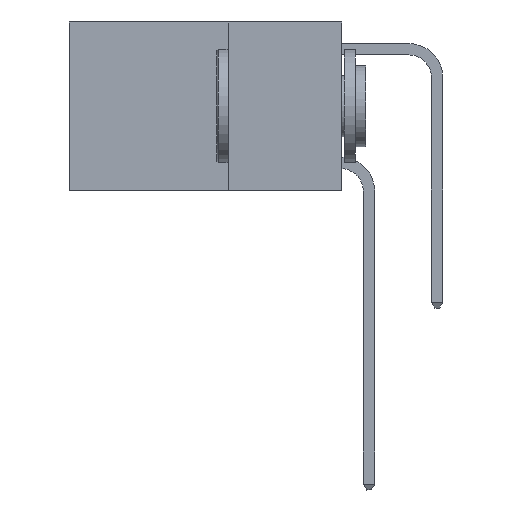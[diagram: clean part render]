
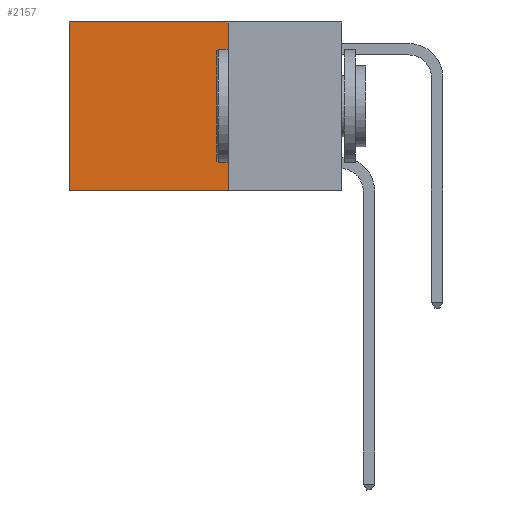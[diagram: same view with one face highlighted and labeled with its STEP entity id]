
A CAD part, left-side view. The second image highlights one B-rep face of the part: STEP entity #2157.
In plain terms, the highlighted planar face has unit normal (-1, 0, 0).
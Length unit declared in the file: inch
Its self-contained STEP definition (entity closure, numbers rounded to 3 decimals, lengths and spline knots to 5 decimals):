
#195 = LINE ( 'NONE', #2769, #5230 ) ;
#414 = ORIENTED_EDGE ( 'NONE', *, *, #4275, .F. ) ;
#1309 = LINE ( 'NONE', #2766, #7239 ) ;
#1412 = DIRECTION ( 'NONE',  ( 0., 0., -1. ) ) ;
#1639 = DIRECTION ( 'NONE',  ( 0., 0., -1. ) ) ;
#1798 = FACE_OUTER_BOUND ( 'NONE', #3617, .T. ) ;
#1962 = DIRECTION ( 'NONE',  ( 0., 0., -1. ) ) ;
#2157 = ADVANCED_FACE ( 'NONE', ( #1798 ), #5561, .F. ) ;
#2766 = CARTESIAN_POINT ( 'NONE',  ( 0.2625, 0.25, -0.37 ) ) ;
#2769 = CARTESIAN_POINT ( 'NONE',  ( 0.2625, 0.25, 0. ) ) ;
#3617 = EDGE_LOOP ( 'NONE', ( #9966, #15439, #414, #15273 ) ) ;
#3849 = VECTOR ( 'NONE', #1412, 39.37008 ) ;
#3919 = EDGE_CURVE ( 'NONE', #5990, #12396, #5336, .T. ) ;
#4057 = DIRECTION ( 'NONE',  ( 0., 1., 0. ) ) ;
#4275 = EDGE_CURVE ( 'NONE', #9997, #16635, #195, .T. ) ;
#5230 = VECTOR ( 'NONE', #1639, 39.37008 ) ;
#5336 = LINE ( 'NONE', #13075, #3849 ) ;
#5561 = PLANE ( 'NONE',  #9439 ) ;
#5988 = CARTESIAN_POINT ( 'NONE',  ( 0.2625, 0.25, 0. ) ) ;
#5990 = VERTEX_POINT ( 'NONE', #6416 ) ;
#6416 = CARTESIAN_POINT ( 'NONE',  ( 0.2625, 0.6, 0. ) ) ;
#7239 = VECTOR ( 'NONE', #14338, 39.37008 ) ;
#9439 = AXIS2_PLACEMENT_3D ( 'NONE', #14915, #9588, #1962 ) ;
#9588 = DIRECTION ( 'NONE',  ( 1., 0., 0. ) ) ;
#9720 = EDGE_CURVE ( 'NONE', #16635, #12396, #1309, .T. ) ;
#9966 = ORIENTED_EDGE ( 'NONE', *, *, #3919, .T. ) ;
#9997 = VERTEX_POINT ( 'NONE', #5988 ) ;
#10397 = CARTESIAN_POINT ( 'NONE',  ( 0.2625, 0.6, -0.37 ) ) ;
#10619 = LINE ( 'NONE', #14685, #11369 ) ;
#11369 = VECTOR ( 'NONE', #4057, 39.37008 ) ;
#12224 = CARTESIAN_POINT ( 'NONE',  ( 0.2625, 0.25, -0.37 ) ) ;
#12396 = VERTEX_POINT ( 'NONE', #10397 ) ;
#12991 = EDGE_CURVE ( 'NONE', #9997, #5990, #10619, .T. ) ;
#13075 = CARTESIAN_POINT ( 'NONE',  ( 0.2625, 0.6, 0. ) ) ;
#14338 = DIRECTION ( 'NONE',  ( 0., 1., 0. ) ) ;
#14685 = CARTESIAN_POINT ( 'NONE',  ( 0.2625, 0.25, 0. ) ) ;
#14915 = CARTESIAN_POINT ( 'NONE',  ( 0.2625, 0.25, 0. ) ) ;
#15273 = ORIENTED_EDGE ( 'NONE', *, *, #12991, .T. ) ;
#15439 = ORIENTED_EDGE ( 'NONE', *, *, #9720, .F. ) ;
#16635 = VERTEX_POINT ( 'NONE', #12224 ) ;
